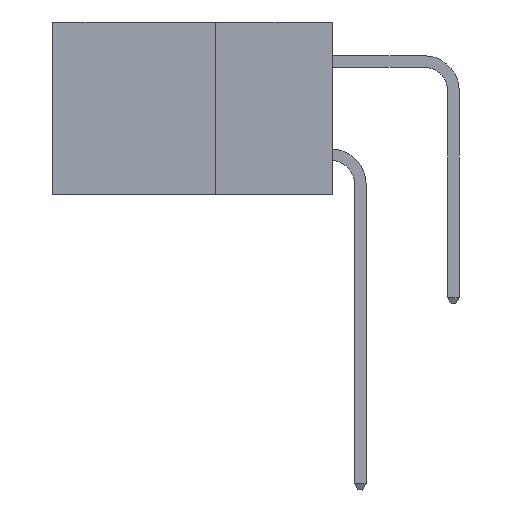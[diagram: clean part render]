
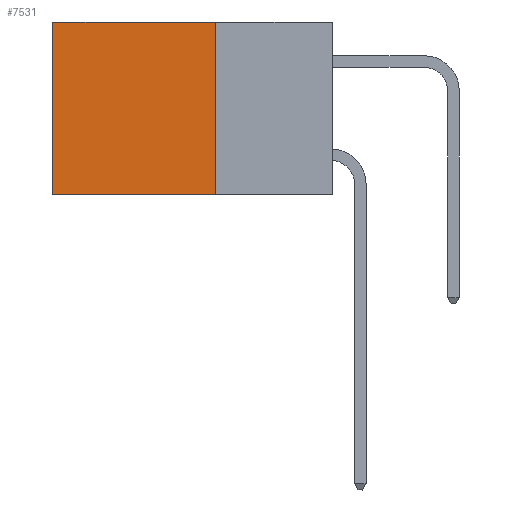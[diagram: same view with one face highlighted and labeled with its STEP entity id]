
A CAD part, left-side view. The second image highlights one B-rep face of the part: STEP entity #7531.
In plain terms, the highlighted planar face has unit normal (-1, 0, 0).
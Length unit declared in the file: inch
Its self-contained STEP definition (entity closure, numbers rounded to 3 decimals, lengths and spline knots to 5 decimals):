
#72 = EDGE_CURVE ( 'NONE', #7662, #14677, #14788, .T. ) ;
#128 = ORIENTED_EDGE ( 'NONE', *, *, #13448, .T. ) ;
#912 = CARTESIAN_POINT ( 'NONE',  ( 0.298, 0.25, -0.37 ) ) ;
#1069 = DIRECTION ( 'NONE',  ( 0., 1., 0. ) ) ;
#1127 = DIRECTION ( 'NONE',  ( 0., 0., -1. ) ) ;
#1553 = VECTOR ( 'NONE', #1127, 39.37008 ) ;
#1647 = EDGE_CURVE ( 'NONE', #7662, #7388, #6583, .T. ) ;
#1990 = LINE ( 'NONE', #17260, #1553 ) ;
#3068 = ORIENTED_EDGE ( 'NONE', *, *, #72, .T. ) ;
#3377 = VECTOR ( 'NONE', #1069, 39.37008 ) ;
#3482 = AXIS2_PLACEMENT_3D ( 'NONE', #4678, #4643, #4637 ) ;
#3774 = CARTESIAN_POINT ( 'NONE',  ( 0.298, 0.25, 0. ) ) ;
#3972 = CARTESIAN_POINT ( 'NONE',  ( 0.298, 0.25, 0. ) ) ;
#4637 = DIRECTION ( 'NONE',  ( 0., 0., -1. ) ) ;
#4643 = DIRECTION ( 'NONE',  ( 1., 0., 0. ) ) ;
#4678 = CARTESIAN_POINT ( 'NONE',  ( 0.298, 0.25, 0. ) ) ;
#4691 = PLANE ( 'NONE',  #3482 ) ;
#6583 = LINE ( 'NONE', #3972, #11079 ) ;
#6614 = CARTESIAN_POINT ( 'NONE',  ( 0.298, 0.25, -0.37 ) ) ;
#6768 = EDGE_CURVE ( 'NONE', #7388, #13865, #10321, .T. ) ;
#7388 = VERTEX_POINT ( 'NONE', #6614 ) ;
#7531 = ADVANCED_FACE ( 'NONE', ( #9245 ), #4691, .F. ) ;
#7662 = VERTEX_POINT ( 'NONE', #3774 ) ;
#7749 = VECTOR ( 'NONE', #12117, 39.37008 ) ;
#9245 = FACE_OUTER_BOUND ( 'NONE', #11733, .T. ) ;
#10282 = ORIENTED_EDGE ( 'NONE', *, *, #6768, .F. ) ;
#10321 = LINE ( 'NONE', #912, #3377 ) ;
#11079 = VECTOR ( 'NONE', #15922, 39.37008 ) ;
#11733 = EDGE_LOOP ( 'NONE', ( #128, #10282, #15374, #3068 ) ) ;
#12117 = DIRECTION ( 'NONE',  ( 0., 1., 0. ) ) ;
#12507 = CARTESIAN_POINT ( 'NONE',  ( 0.298, 0.25, 0. ) ) ;
#13448 = EDGE_CURVE ( 'NONE', #14677, #13865, #1990, .T. ) ;
#13865 = VERTEX_POINT ( 'NONE', #16816 ) ;
#14043 = CARTESIAN_POINT ( 'NONE',  ( 0.298, 0.6, 0. ) ) ;
#14677 = VERTEX_POINT ( 'NONE', #14043 ) ;
#14788 = LINE ( 'NONE', #12507, #7749 ) ;
#15374 = ORIENTED_EDGE ( 'NONE', *, *, #1647, .F. ) ;
#15922 = DIRECTION ( 'NONE',  ( 0., 0., -1. ) ) ;
#16816 = CARTESIAN_POINT ( 'NONE',  ( 0.298, 0.6, -0.37 ) ) ;
#17260 = CARTESIAN_POINT ( 'NONE',  ( 0.298, 0.6, 0. ) ) ;
